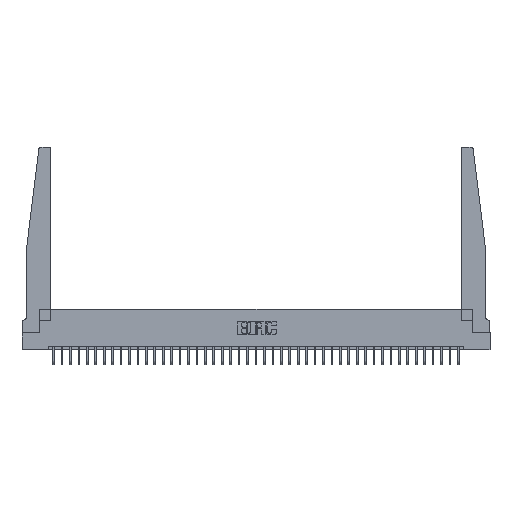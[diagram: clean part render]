
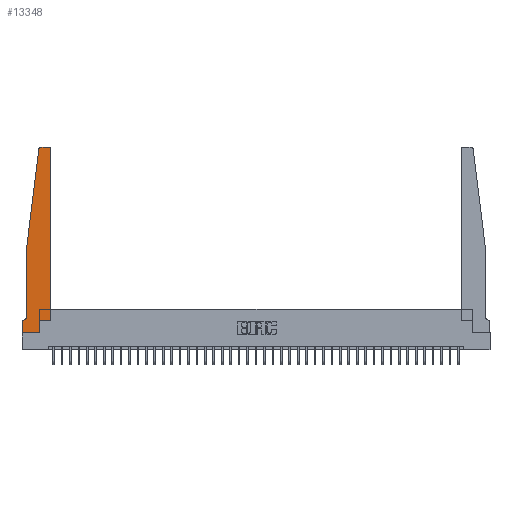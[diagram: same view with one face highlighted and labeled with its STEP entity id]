
A CAD part, top view. The second image highlights one B-rep face of the part: STEP entity #13348.
In plain terms, the highlighted planar face has unit normal (0, 0, 1).
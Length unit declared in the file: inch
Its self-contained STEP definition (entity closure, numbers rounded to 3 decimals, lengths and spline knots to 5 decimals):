
#418 = ORIENTED_EDGE ( 'NONE', *, *, #33483, .T. ) ;
#446 = CARTESIAN_POINT ( 'NONE',  ( 0.425, 0.18, 0.37 ) ) ;
#688 = DIRECTION ( 'NONE',  ( 1., 0., 0. ) ) ;
#1290 = CARTESIAN_POINT ( 'NONE',  ( 0.395, 2.75, 0.37 ) ) ;
#1391 = VERTEX_POINT ( 'NONE', #1290 ) ;
#2058 = CARTESIAN_POINT ( 'NONE',  ( 0., 0., 0.37 ) ) ;
#2098 = VECTOR ( 'NONE', #31160, 39.37008 ) ;
#2195 = CARTESIAN_POINT ( 'NONE',  ( 0.395, 2.72, 0.37 ) ) ;
#2498 = ORIENTED_EDGE ( 'NONE', *, *, #15431, .T. ) ;
#2499 = ORIENTED_EDGE ( 'NONE', *, *, #4930, .T. ) ;
#3003 = EDGE_CURVE ( 'NONE', #1391, #32191, #7367, .T. ) ;
#3596 = ORIENTED_EDGE ( 'NONE', *, *, #28448, .T. ) ;
#4637 = CARTESIAN_POINT ( 'NONE',  ( 0.065, 1.25, 0.37 ) ) ;
#4770 = VERTEX_POINT ( 'NONE', #18714 ) ;
#4930 = EDGE_CURVE ( 'NONE', #36509, #22460, #26858, .T. ) ;
#5094 = CARTESIAN_POINT ( 'NONE',  ( 0.065, 1.25, 0.37 ) ) ;
#5125 = DIRECTION ( 'NONE',  ( 0., 0., 1. ) ) ;
#6248 = VERTEX_POINT ( 'NONE', #10484 ) ;
#6307 = EDGE_CURVE ( 'NONE', #22460, #1391, #32617, .T. ) ;
#6447 = DIRECTION ( 'NONE',  ( 0., 1., 0. ) ) ;
#7367 = LINE ( 'NONE', #36751, #24650 ) ;
#7611 = CARTESIAN_POINT ( 'NONE',  ( 0.27653, 2.75, 0.37 ) ) ;
#7666 = CARTESIAN_POINT ( 'NONE',  ( 0.425, 0.18, 0.37 ) ) ;
#7720 = LINE ( 'NONE', #33813, #22265 ) ;
#7978 = EDGE_CURVE ( 'NONE', #11571, #4770, #16262, .T. ) ;
#8209 = DIRECTION ( 'NONE',  ( 1., 0., 0. ) ) ;
#9019 = EDGE_CURVE ( 'NONE', #6248, #12104, #18895, .T. ) ;
#9952 = EDGE_CURVE ( 'NONE', #4770, #28845, #35632, .T. ) ;
#10484 = CARTESIAN_POINT ( 'NONE',  ( 0.24675, 2.72367, 0.37 ) ) ;
#11571 = VERTEX_POINT ( 'NONE', #26352 ) ;
#12104 = VERTEX_POINT ( 'NONE', #15818 ) ;
#12253 = ORIENTED_EDGE ( 'NONE', *, *, #6307, .T. ) ;
#12562 = VERTEX_POINT ( 'NONE', #35851 ) ;
#12796 = CIRCLE ( 'NONE', #29811, 0.05 ) ;
#13348 = ADVANCED_FACE ( 'NONE', ( #34954 ), #13769, .T. ) ;
#13625 = CIRCLE ( 'NONE', #26818, 0.03 ) ;
#13769 = PLANE ( 'NONE',  #16796 ) ;
#13776 = DIRECTION ( 'NONE',  ( 0., -1., 0. ) ) ;
#14833 = EDGE_CURVE ( 'NONE', #12562, #11571, #7720, .T. ) ;
#15431 = EDGE_CURVE ( 'NONE', #32191, #6248, #13625, .T. ) ;
#15708 = CARTESIAN_POINT ( 'NONE',  ( 0.2605, 0.18, 0.37 ) ) ;
#15818 = CARTESIAN_POINT ( 'NONE',  ( 0.065, 1.25, 0.37 ) ) ;
#15905 = LINE ( 'NONE', #446, #23699 ) ;
#16177 = CARTESIAN_POINT ( 'NONE',  ( 0.015, 0.1875, 0.37 ) ) ;
#16262 = LINE ( 'NONE', #2058, #24453 ) ;
#16796 = AXIS2_PLACEMENT_3D ( 'NONE', #34910, #17398, #26213 ) ;
#17398 = DIRECTION ( 'NONE',  ( 0., 0., 1. ) ) ;
#17628 = DIRECTION ( 'NONE',  ( -1., 0., 0. ) ) ;
#17764 = ORIENTED_EDGE ( 'NONE', *, *, #7978, .T. ) ;
#18714 = CARTESIAN_POINT ( 'NONE',  ( 0.2605, 0., 0.37 ) ) ;
#18811 = VECTOR ( 'NONE', #20811, 39.37008 ) ;
#18895 = LINE ( 'NONE', #4637, #33907 ) ;
#19248 = DIRECTION ( 'NONE',  ( -0.122, -0.992, 0. ) ) ;
#19282 = LINE ( 'NONE', #26675, #18811 ) ;
#19538 = EDGE_LOOP ( 'NONE', ( #35949, #2498, #35404, #418, #24421, #3596, #25477, #17764, #33286, #33434, #2499, #12253 ) ) ;
#19638 = VERTEX_POINT ( 'NONE', #28039 ) ;
#20424 = DIRECTION ( 'NONE',  ( 0., 0., -1. ) ) ;
#20811 = DIRECTION ( 'NONE',  ( -1., 0., 0. ) ) ;
#22265 = VECTOR ( 'NONE', #13776, 39.37008 ) ;
#22460 = VERTEX_POINT ( 'NONE', #26808 ) ;
#22860 = DIRECTION ( 'NONE',  ( -1., 0., 0. ) ) ;
#23466 = CARTESIAN_POINT ( 'NONE',  ( 0.425, 0.18, 0.37 ) ) ;
#23699 = VECTOR ( 'NONE', #688, 39.37008 ) ;
#24421 = ORIENTED_EDGE ( 'NONE', *, *, #30835, .T. ) ;
#24453 = VECTOR ( 'NONE', #33709, 39.37008 ) ;
#24650 = VECTOR ( 'NONE', #17628, 39.37008 ) ;
#24658 = DIRECTION ( 'NONE',  ( 0., 0., 1. ) ) ;
#24798 = DIRECTION ( 'NONE',  ( 1., 0., 0. ) ) ;
#25477 = ORIENTED_EDGE ( 'NONE', *, *, #14833, .T. ) ;
#26213 = DIRECTION ( 'NONE',  ( 1., 0., 0. ) ) ;
#26352 = CARTESIAN_POINT ( 'NONE',  ( 0., 0., 0.37 ) ) ;
#26675 = CARTESIAN_POINT ( 'NONE',  ( 0.065, 0.1875, 0.37 ) ) ;
#26781 = EDGE_CURVE ( 'NONE', #28845, #36509, #15905, .T. ) ;
#26808 = CARTESIAN_POINT ( 'NONE',  ( 0.425, 2.72, 0.37 ) ) ;
#26818 = AXIS2_PLACEMENT_3D ( 'NONE', #30739, #24658, #24798 ) ;
#26858 = LINE ( 'NONE', #7666, #29591 ) ;
#27996 = VECTOR ( 'NONE', #6447, 39.37008 ) ;
#28039 = CARTESIAN_POINT ( 'NONE',  ( 0.065, 0.2375, 0.37 ) ) ;
#28448 = EDGE_CURVE ( 'NONE', #29428, #12562, #19282, .T. ) ;
#28845 = VERTEX_POINT ( 'NONE', #15708 ) ;
#29428 = VERTEX_POINT ( 'NONE', #16177 ) ;
#29591 = VECTOR ( 'NONE', #33801, 39.37008 ) ;
#29811 = AXIS2_PLACEMENT_3D ( 'NONE', #31610, #20424, #22860 ) ;
#30739 = CARTESIAN_POINT ( 'NONE',  ( 0.27653, 2.72, 0.37 ) ) ;
#30835 = EDGE_CURVE ( 'NONE', #19638, #29428, #12796, .T. ) ;
#31160 = DIRECTION ( 'NONE',  ( 0., -1., 0. ) ) ;
#31610 = CARTESIAN_POINT ( 'NONE',  ( 0.015, 0.2375, 0.37 ) ) ;
#32191 = VERTEX_POINT ( 'NONE', #7611 ) ;
#32617 = CIRCLE ( 'NONE', #34646, 0.03 ) ;
#33286 = ORIENTED_EDGE ( 'NONE', *, *, #9952, .T. ) ;
#33434 = ORIENTED_EDGE ( 'NONE', *, *, #26781, .T. ) ;
#33483 = EDGE_CURVE ( 'NONE', #12104, #19638, #35718, .T. ) ;
#33709 = DIRECTION ( 'NONE',  ( 1., 0., 0. ) ) ;
#33801 = DIRECTION ( 'NONE',  ( 0., 1., 0. ) ) ;
#33813 = CARTESIAN_POINT ( 'NONE',  ( 0., 0., 0.37 ) ) ;
#33907 = VECTOR ( 'NONE', #19248, 39.37008 ) ;
#34646 = AXIS2_PLACEMENT_3D ( 'NONE', #2195, #5125, #8209 ) ;
#34910 = CARTESIAN_POINT ( 'NONE',  ( 0., 0.1875, 0.37 ) ) ;
#34954 = FACE_OUTER_BOUND ( 'NONE', #19538, .T. ) ;
#35023 = CARTESIAN_POINT ( 'NONE',  ( 0.2605, 0.18, 0.37 ) ) ;
#35404 = ORIENTED_EDGE ( 'NONE', *, *, #9019, .T. ) ;
#35632 = LINE ( 'NONE', #35023, #27996 ) ;
#35718 = LINE ( 'NONE', #5094, #2098 ) ;
#35851 = CARTESIAN_POINT ( 'NONE',  ( 0., 0.1875, 0.37 ) ) ;
#35949 = ORIENTED_EDGE ( 'NONE', *, *, #3003, .T. ) ;
#36509 = VERTEX_POINT ( 'NONE', #23466 ) ;
#36751 = CARTESIAN_POINT ( 'NONE',  ( 0.25, 2.75, 0.37 ) ) ;
